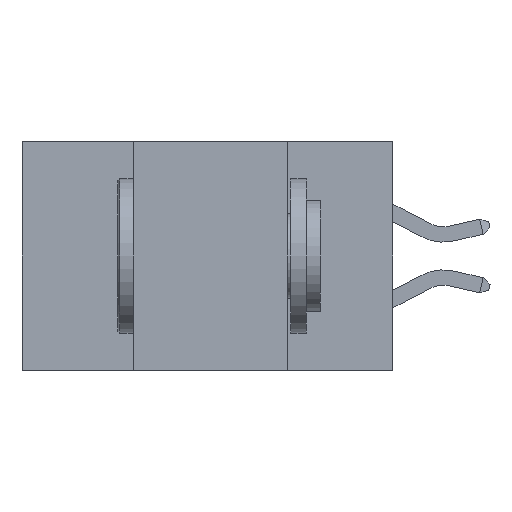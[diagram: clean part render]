
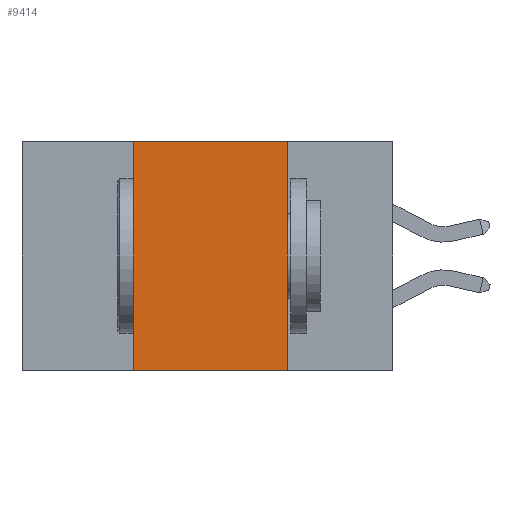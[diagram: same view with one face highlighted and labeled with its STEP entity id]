
A CAD part, left-side view. The second image highlights one B-rep face of the part: STEP entity #9414.
In plain terms, the highlighted planar face has unit normal (-1, 0, 0).
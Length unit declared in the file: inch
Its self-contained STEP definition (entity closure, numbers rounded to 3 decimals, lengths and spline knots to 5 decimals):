
#464 = VERTEX_POINT ( 'NONE', #12998 ) ;
#2760 = CARTESIAN_POINT ( 'NONE',  ( 0., 0.6, 0. ) ) ;
#2966 = EDGE_LOOP ( 'NONE', ( #13325, #12896, #11598, #6955 ) ) ;
#3620 = VERTEX_POINT ( 'NONE', #10821 ) ;
#3781 = VERTEX_POINT ( 'NONE', #7312 ) ;
#4267 = DIRECTION ( 'NONE',  ( 0., 0., -1. ) ) ;
#4347 = AXIS2_PLACEMENT_3D ( 'NONE', #2760, #12696, #4267 ) ;
#4548 = VECTOR ( 'NONE', #13067, 39.37008 ) ;
#4696 = EDGE_CURVE ( 'NONE', #3781, #7095, #15702, .T. ) ;
#5060 = EDGE_CURVE ( 'NONE', #464, #7095, #16789, .T. ) ;
#5147 = VECTOR ( 'NONE', #13587, 39.37008 ) ;
#6472 = CARTESIAN_POINT ( 'NONE',  ( 0., 0.42, 0. ) ) ;
#6955 = ORIENTED_EDGE ( 'NONE', *, *, #4696, .T. ) ;
#7095 = VERTEX_POINT ( 'NONE', #9736 ) ;
#7312 = CARTESIAN_POINT ( 'NONE',  ( 0., 0.42, -0.37 ) ) ;
#8914 = LINE ( 'NONE', #17758, #5147 ) ;
#9414 = ADVANCED_FACE ( 'NONE', ( #16709 ), #11317, .F. ) ;
#9472 = VECTOR ( 'NONE', #9742, 39.37008 ) ;
#9736 = CARTESIAN_POINT ( 'NONE',  ( 0., 0.17, -0.37 ) ) ;
#9742 = DIRECTION ( 'NONE',  ( 0., 0., -1. ) ) ;
#9813 = EDGE_CURVE ( 'NONE', #3781, #3620, #17125, .T. ) ;
#9890 = EDGE_CURVE ( 'NONE', #3620, #464, #8914, .T. ) ;
#10821 = CARTESIAN_POINT ( 'NONE',  ( 0., 0.42, 0. ) ) ;
#11317 = PLANE ( 'NONE',  #4347 ) ;
#11598 = ORIENTED_EDGE ( 'NONE', *, *, #9813, .F. ) ;
#12696 = DIRECTION ( 'NONE',  ( 1., 0., 0. ) ) ;
#12896 = ORIENTED_EDGE ( 'NONE', *, *, #9890, .F. ) ;
#12998 = CARTESIAN_POINT ( 'NONE',  ( 0., 0.17, 0. ) ) ;
#13067 = DIRECTION ( 'NONE',  ( 0., -1., 0. ) ) ;
#13325 = ORIENTED_EDGE ( 'NONE', *, *, #5060, .F. ) ;
#13460 = DIRECTION ( 'NONE',  ( 0., 0., 1. ) ) ;
#13587 = DIRECTION ( 'NONE',  ( 0., -1., 0. ) ) ;
#15702 = LINE ( 'NONE', #17155, #4548 ) ;
#16597 = CARTESIAN_POINT ( 'NONE',  ( 0., 0.17, 0. ) ) ;
#16691 = VECTOR ( 'NONE', #13460, 39.37008 ) ;
#16709 = FACE_OUTER_BOUND ( 'NONE', #2966, .T. ) ;
#16789 = LINE ( 'NONE', #16597, #9472 ) ;
#17125 = LINE ( 'NONE', #6472, #16691 ) ;
#17155 = CARTESIAN_POINT ( 'NONE',  ( 0., 0.6, -0.37 ) ) ;
#17758 = CARTESIAN_POINT ( 'NONE',  ( 0., 0.6, 0. ) ) ;
